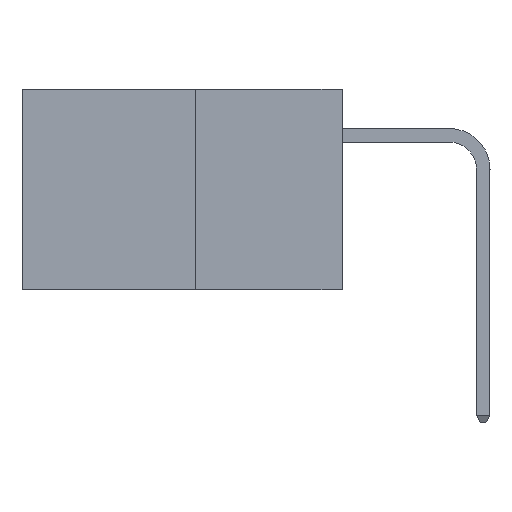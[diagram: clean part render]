
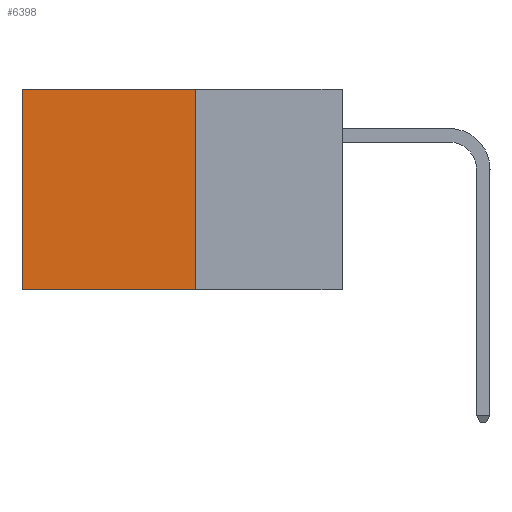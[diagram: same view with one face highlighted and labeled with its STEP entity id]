
A CAD part, left-side view. The second image highlights one B-rep face of the part: STEP entity #6398.
In plain terms, the highlighted planar face has unit normal (-1, 0, 0).
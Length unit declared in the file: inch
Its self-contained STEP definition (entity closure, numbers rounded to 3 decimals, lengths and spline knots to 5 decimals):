
#222 = VECTOR ( 'NONE', #14536, 39.37008 ) ;
#1080 = PLANE ( 'NONE',  #14798 ) ;
#1582 = VERTEX_POINT ( 'NONE', #15937 ) ;
#1844 = ORIENTED_EDGE ( 'NONE', *, *, #6543, .T. ) ;
#3301 = CARTESIAN_POINT ( 'NONE',  ( 0.277, 0.27, 0. ) ) ;
#3940 = CARTESIAN_POINT ( 'NONE',  ( 0.277, 0.59, -0.37 ) ) ;
#4184 = DIRECTION ( 'NONE',  ( 1., 0., 0. ) ) ;
#5377 = VECTOR ( 'NONE', #19124, 39.37008 ) ;
#6000 = DIRECTION ( 'NONE',  ( 0., 0., -1. ) ) ;
#6398 = ADVANCED_FACE ( 'NONE', ( #11505 ), #1080, .F. ) ;
#6543 = EDGE_CURVE ( 'NONE', #19216, #17027, #9042, .T. ) ;
#6567 = ORIENTED_EDGE ( 'NONE', *, *, #7195, .F. ) ;
#6732 = EDGE_LOOP ( 'NONE', ( #1844, #18366, #6567, #11416 ) ) ;
#7195 = EDGE_CURVE ( 'NONE', #19722, #1582, #16881, .T. ) ;
#7927 = LINE ( 'NONE', #13025, #222 ) ;
#8225 = CARTESIAN_POINT ( 'NONE',  ( 0.277, 0.27, -0.37 ) ) ;
#8724 = CARTESIAN_POINT ( 'NONE',  ( 0.277, 0.27, -0.37 ) ) ;
#9042 = LINE ( 'NONE', #15408, #12733 ) ;
#9818 = EDGE_CURVE ( 'NONE', #19722, #19216, #7927, .T. ) ;
#10032 = LINE ( 'NONE', #8724, #14226 ) ;
#11416 = ORIENTED_EDGE ( 'NONE', *, *, #9818, .T. ) ;
#11505 = FACE_OUTER_BOUND ( 'NONE', #6732, .T. ) ;
#12733 = VECTOR ( 'NONE', #6000, 39.37008 ) ;
#13025 = CARTESIAN_POINT ( 'NONE',  ( 0.277, 0.27, 0. ) ) ;
#13479 = CARTESIAN_POINT ( 'NONE',  ( 0.277, 0.27, -0.37 ) ) ;
#14226 = VECTOR ( 'NONE', #19620, 39.37008 ) ;
#14391 = CARTESIAN_POINT ( 'NONE',  ( 0.277, 0.59, 0. ) ) ;
#14536 = DIRECTION ( 'NONE',  ( 0., 1., 0. ) ) ;
#14747 = EDGE_CURVE ( 'NONE', #1582, #17027, #10032, .T. ) ;
#14798 = AXIS2_PLACEMENT_3D ( 'NONE', #13479, #4184, #15139 ) ;
#15139 = DIRECTION ( 'NONE',  ( 0., 0., -1. ) ) ;
#15408 = CARTESIAN_POINT ( 'NONE',  ( 0.277, 0.59, -0.37 ) ) ;
#15937 = CARTESIAN_POINT ( 'NONE',  ( 0.277, 0.27, -0.37 ) ) ;
#16881 = LINE ( 'NONE', #8225, #5377 ) ;
#17027 = VERTEX_POINT ( 'NONE', #3940 ) ;
#18366 = ORIENTED_EDGE ( 'NONE', *, *, #14747, .F. ) ;
#19124 = DIRECTION ( 'NONE',  ( 0., 0., -1. ) ) ;
#19216 = VERTEX_POINT ( 'NONE', #14391 ) ;
#19620 = DIRECTION ( 'NONE',  ( 0., 1., 0. ) ) ;
#19722 = VERTEX_POINT ( 'NONE', #3301 ) ;
